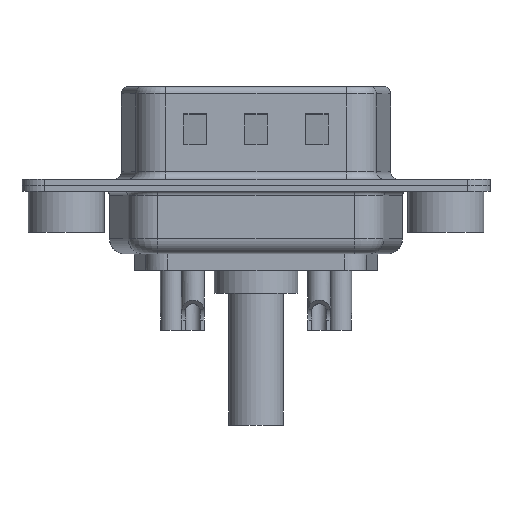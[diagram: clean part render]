
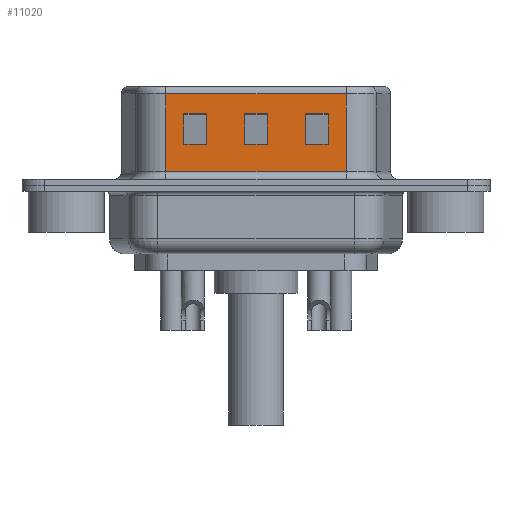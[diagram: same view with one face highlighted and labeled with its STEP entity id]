
A CAD part, front view. The second image highlights one B-rep face of the part: STEP entity #11020.
In plain terms, the highlighted planar face has unit normal (0, -1, 0).
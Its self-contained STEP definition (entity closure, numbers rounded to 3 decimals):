
#124 = PLANE ( 'NONE',  #6865 ) ;
#260 = VERTEX_POINT ( 'NONE', #16972 ) ;
#380 = VERTEX_POINT ( 'NONE', #1488 ) ;
#493 = VECTOR ( 'NONE', #16923, 1000. ) ;
#636 = VERTEX_POINT ( 'NONE', #8105 ) ;
#662 = LINE ( 'NONE', #11639, #13870 ) ;
#691 = CARTESIAN_POINT ( 'NONE',  ( 13.25, -4.58, 4.705 ) ) ;
#714 = ORIENTED_EDGE ( 'NONE', *, *, #1683, .F. ) ;
#862 = EDGE_CURVE ( 'NONE', #14935, #6580, #16073, .T. ) ;
#940 = LINE ( 'NONE', #13751, #14536 ) ;
#989 = EDGE_LOOP ( 'NONE', ( #11860, #16976, #4822, #14950 ) ) ;
#1067 = CARTESIAN_POINT ( 'NONE',  ( 15.75, -4.58, 2.705 ) ) ;
#1095 = CARTESIAN_POINT ( 'NONE',  ( 11.75, -4.58, 6.52 ) ) ;
#1154 = DIRECTION ( 'NONE',  ( 0., 0., -1. ) ) ;
#1307 = EDGE_CURVE ( 'NONE', #260, #636, #7129, .T. ) ;
#1400 = ORIENTED_EDGE ( 'NONE', *, *, #1307, .T. ) ;
#1488 = CARTESIAN_POINT ( 'NONE',  ( 17.25, -4.58, 2.705 ) ) ;
#1501 = VECTOR ( 'NONE', #5160, 1000. ) ;
#1532 = DIRECTION ( 'NONE',  ( 0., 0., 1. ) ) ;
#1683 = EDGE_CURVE ( 'NONE', #6942, #7835, #9648, .T. ) ;
#2054 = VECTOR ( 'NONE', #11375, 1000. ) ;
#2211 = FACE_OUTER_BOUND ( 'NONE', #14918, .T. ) ;
#2329 = LINE ( 'NONE', #7532, #1501 ) ;
#2668 = VECTOR ( 'NONE', #6847, 1000. ) ;
#2717 = CARTESIAN_POINT ( 'NONE',  ( 14.45, -4.58, 4.705 ) ) ;
#2728 = LINE ( 'NONE', #10076, #16320 ) ;
#2823 = ORIENTED_EDGE ( 'NONE', *, *, #15987, .T. ) ;
#2976 = DIRECTION ( 'NONE',  ( -1., 0., 0. ) ) ;
#3106 = ORIENTED_EDGE ( 'NONE', *, *, #9867, .T. ) ;
#3187 = DIRECTION ( 'NONE',  ( 0., 0., -1. ) ) ;
#3507 = CARTESIAN_POINT ( 'NONE',  ( 18.45, -4.58, 6.52 ) ) ;
#3695 = VERTEX_POINT ( 'NONE', #4711 ) ;
#3773 = EDGE_CURVE ( 'NONE', #7875, #7835, #13329, .T. ) ;
#3916 = CARTESIAN_POINT ( 'NONE',  ( 15.75, -4.58, 6.52 ) ) ;
#4045 = CARTESIAN_POINT ( 'NONE',  ( 22.45, -4.58, 2.705 ) ) ;
#4268 = EDGE_CURVE ( 'NONE', #7696, #7875, #940, .T. ) ;
#4606 = LINE ( 'NONE', #16934, #7682 ) ;
#4711 = CARTESIAN_POINT ( 'NONE',  ( 17.25, -4.58, 4.705 ) ) ;
#4718 = DIRECTION ( 'NONE',  ( 1., 0., 0. ) ) ;
#4822 = ORIENTED_EDGE ( 'NONE', *, *, #8445, .T. ) ;
#5028 = CARTESIAN_POINT ( 'NONE',  ( 18.45, -4.58, 4.705 ) ) ;
#5057 = CARTESIAN_POINT ( 'NONE',  ( 13.25, -4.58, 2.705 ) ) ;
#5160 = DIRECTION ( 'NONE',  ( 1., 0., 0. ) ) ;
#5290 = DIRECTION ( 'NONE',  ( -1., 0., 0. ) ) ;
#5330 = LINE ( 'NONE', #4045, #11634 ) ;
#5516 = VECTOR ( 'NONE', #10310, 1000. ) ;
#5607 = FACE_BOUND ( 'NONE', #13853, .T. ) ;
#5804 = ORIENTED_EDGE ( 'NONE', *, *, #5927, .T. ) ;
#5823 = EDGE_CURVE ( 'NONE', #380, #10790, #5330, .T. ) ;
#5859 = VECTOR ( 'NONE', #3187, 1000. ) ;
#5927 = EDGE_CURVE ( 'NONE', #15699, #10583, #662, .T. ) ;
#6028 = FACE_BOUND ( 'NONE', #989, .T. ) ;
#6038 = CARTESIAN_POINT ( 'NONE',  ( 11.75, -4.58, 2.705 ) ) ;
#6420 = EDGE_CURVE ( 'NONE', #9559, #3695, #2329, .T. ) ;
#6580 = VERTEX_POINT ( 'NONE', #691 ) ;
#6847 = DIRECTION ( 'NONE',  ( 0., 0., -1. ) ) ;
#6865 = AXIS2_PLACEMENT_3D ( 'NONE', #13352, #9402, #1532 ) ;
#6942 = VERTEX_POINT ( 'NONE', #9698 ) ;
#6970 = DIRECTION ( 'NONE',  ( 0., 0., -1. ) ) ;
#7129 = LINE ( 'NONE', #2717, #13782 ) ;
#7233 = LINE ( 'NONE', #3916, #10390 ) ;
#7532 = CARTESIAN_POINT ( 'NONE',  ( 22.45, -4.58, 4.705 ) ) ;
#7540 = LINE ( 'NONE', #13296, #11533 ) ;
#7682 = VECTOR ( 'NONE', #1154, 1000. ) ;
#7696 = VERTEX_POINT ( 'NONE', #15601 ) ;
#7835 = VERTEX_POINT ( 'NONE', #9339 ) ;
#7875 = VERTEX_POINT ( 'NONE', #12098 ) ;
#8105 = CARTESIAN_POINT ( 'NONE',  ( 9.25, -4.58, 4.705 ) ) ;
#8413 = LINE ( 'NONE', #10691, #11568 ) ;
#8445 = EDGE_CURVE ( 'NONE', #13668, #15488, #8413, .T. ) ;
#8652 = EDGE_CURVE ( 'NONE', #636, #15699, #9462, .T. ) ;
#9198 = FACE_BOUND ( 'NONE', #14284, .T. ) ;
#9339 = CARTESIAN_POINT ( 'NONE',  ( 18.45, -4.58, 0.9 ) ) ;
#9402 = DIRECTION ( 'NONE',  ( 0., 1., 0. ) ) ;
#9462 = LINE ( 'NONE', #16310, #5859 ) ;
#9559 = VERTEX_POINT ( 'NONE', #15312 ) ;
#9648 = LINE ( 'NONE', #3507, #2668 ) ;
#9698 = CARTESIAN_POINT ( 'NONE',  ( 18.45, -4.58, 6.02 ) ) ;
#9867 = EDGE_CURVE ( 'NONE', #6942, #7696, #7540, .T. ) ;
#10023 = ORIENTED_EDGE ( 'NONE', *, *, #6420, .T. ) ;
#10076 = CARTESIAN_POINT ( 'NONE',  ( 7.75, -4.58, 6.52 ) ) ;
#10117 = VECTOR ( 'NONE', #6970, 1000. ) ;
#10310 = DIRECTION ( 'NONE',  ( 0., 0., 1. ) ) ;
#10390 = VECTOR ( 'NONE', #11802, 1000. ) ;
#10583 = VERTEX_POINT ( 'NONE', #10735 ) ;
#10691 = CARTESIAN_POINT ( 'NONE',  ( 18.45, -4.58, 2.705 ) ) ;
#10735 = CARTESIAN_POINT ( 'NONE',  ( 7.75, -4.58, 2.705 ) ) ;
#10790 = VERTEX_POINT ( 'NONE', #1067 ) ;
#11020 = ADVANCED_FACE ( 'NONE', ( #5607, #9198, #6028, #2211 ), #124, .F. ) ;
#11375 = DIRECTION ( 'NONE',  ( 1., 0., 0. ) ) ;
#11389 = CARTESIAN_POINT ( 'NONE',  ( 18.45, -4.58, 0.9 ) ) ;
#11412 = DIRECTION ( 'NONE',  ( 0., 0., -1. ) ) ;
#11533 = VECTOR ( 'NONE', #5290, 1000. ) ;
#11568 = VECTOR ( 'NONE', #12026, 1000. ) ;
#11634 = VECTOR ( 'NONE', #12301, 1000. ) ;
#11639 = CARTESIAN_POINT ( 'NONE',  ( 14.45, -4.58, 2.705 ) ) ;
#11802 = DIRECTION ( 'NONE',  ( 0., 0., 1. ) ) ;
#11860 = ORIENTED_EDGE ( 'NONE', *, *, #862, .T. ) ;
#12026 = DIRECTION ( 'NONE',  ( -1., 0., 0. ) ) ;
#12098 = CARTESIAN_POINT ( 'NONE',  ( 6.55, -4.58, 0.9 ) ) ;
#12301 = DIRECTION ( 'NONE',  ( -1., 0., 0. ) ) ;
#12371 = EDGE_CURVE ( 'NONE', #6580, #13668, #4606, .T. ) ;
#13030 = EDGE_CURVE ( 'NONE', #10790, #9559, #7233, .T. ) ;
#13240 = CARTESIAN_POINT ( 'NONE',  ( 9.25, -4.58, 2.705 ) ) ;
#13296 = CARTESIAN_POINT ( 'NONE',  ( 18.45, -4.58, 6.02 ) ) ;
#13329 = LINE ( 'NONE', #11389, #493 ) ;
#13352 = CARTESIAN_POINT ( 'NONE',  ( 18.45, -4.58, 6.52 ) ) ;
#13658 = CARTESIAN_POINT ( 'NONE',  ( 17.25, -4.58, 6.52 ) ) ;
#13668 = VERTEX_POINT ( 'NONE', #5057 ) ;
#13751 = CARTESIAN_POINT ( 'NONE',  ( 6.55, -4.58, 6.52 ) ) ;
#13782 = VECTOR ( 'NONE', #4718, 1000. ) ;
#13853 = EDGE_LOOP ( 'NONE', ( #15978, #5804, #16044, #1400 ) ) ;
#13870 = VECTOR ( 'NONE', #2976, 1000. ) ;
#14056 = DIRECTION ( 'NONE',  ( 0., 0., 1. ) ) ;
#14059 = ORIENTED_EDGE ( 'NONE', *, *, #13030, .T. ) ;
#14284 = EDGE_LOOP ( 'NONE', ( #2823, #16307, #14059, #10023 ) ) ;
#14536 = VECTOR ( 'NONE', #11412, 1000. ) ;
#14542 = EDGE_CURVE ( 'NONE', #10583, #260, #2728, .T. ) ;
#14647 = EDGE_CURVE ( 'NONE', #15488, #14935, #15744, .T. ) ;
#14724 = CARTESIAN_POINT ( 'NONE',  ( 11.75, -4.58, 4.705 ) ) ;
#14764 = ORIENTED_EDGE ( 'NONE', *, *, #4268, .T. ) ;
#14781 = ORIENTED_EDGE ( 'NONE', *, *, #3773, .T. ) ;
#14918 = EDGE_LOOP ( 'NONE', ( #714, #3106, #14764, #14781 ) ) ;
#14935 = VERTEX_POINT ( 'NONE', #14724 ) ;
#14950 = ORIENTED_EDGE ( 'NONE', *, *, #14647, .T. ) ;
#15312 = CARTESIAN_POINT ( 'NONE',  ( 15.75, -4.58, 4.705 ) ) ;
#15488 = VERTEX_POINT ( 'NONE', #6038 ) ;
#15601 = CARTESIAN_POINT ( 'NONE',  ( 6.55, -4.58, 6.02 ) ) ;
#15699 = VERTEX_POINT ( 'NONE', #13240 ) ;
#15744 = LINE ( 'NONE', #1095, #5516 ) ;
#15978 = ORIENTED_EDGE ( 'NONE', *, *, #8652, .T. ) ;
#15987 = EDGE_CURVE ( 'NONE', #3695, #380, #17138, .T. ) ;
#16044 = ORIENTED_EDGE ( 'NONE', *, *, #14542, .T. ) ;
#16073 = LINE ( 'NONE', #5028, #2054 ) ;
#16307 = ORIENTED_EDGE ( 'NONE', *, *, #5823, .T. ) ;
#16310 = CARTESIAN_POINT ( 'NONE',  ( 9.25, -4.58, 6.52 ) ) ;
#16320 = VECTOR ( 'NONE', #14056, 1000. ) ;
#16923 = DIRECTION ( 'NONE',  ( 1., 0., 0. ) ) ;
#16934 = CARTESIAN_POINT ( 'NONE',  ( 13.25, -4.58, 6.52 ) ) ;
#16972 = CARTESIAN_POINT ( 'NONE',  ( 7.75, -4.58, 4.705 ) ) ;
#16976 = ORIENTED_EDGE ( 'NONE', *, *, #12371, .T. ) ;
#17138 = LINE ( 'NONE', #13658, #10117 ) ;
